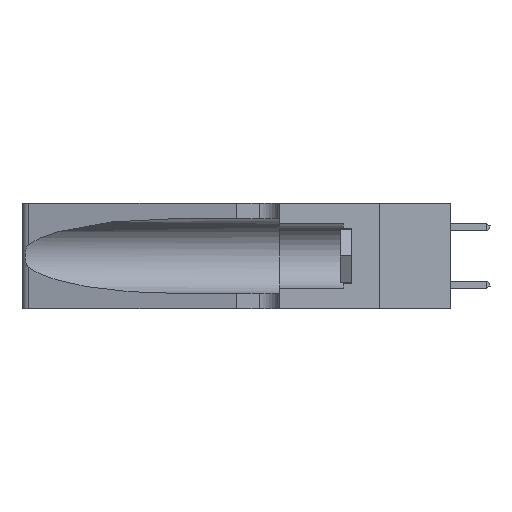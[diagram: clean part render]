
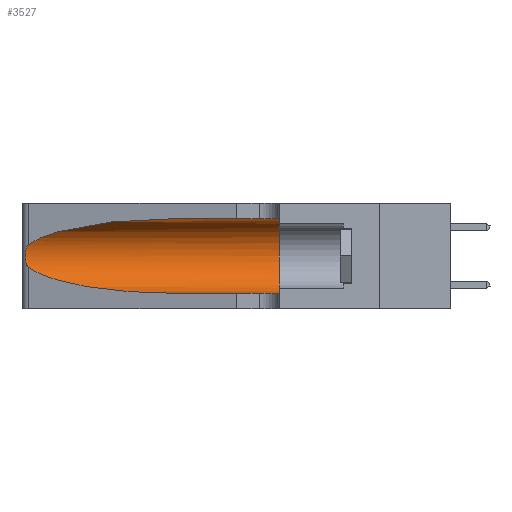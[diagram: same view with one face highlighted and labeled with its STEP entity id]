
A CAD part, left-side view. The second image highlights one B-rep face of the part: STEP entity #3527.
In plain terms, the highlighted cylindrical face has radius 3.308 mm (diameter 6.617 mm), a partial arc.
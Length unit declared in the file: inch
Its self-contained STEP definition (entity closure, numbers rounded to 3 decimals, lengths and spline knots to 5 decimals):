
#515 = EDGE_CURVE ( 'NONE', #18093, #35424, #3145, .T. ) ;
#1190 = ORIENTED_EDGE ( 'NONE', *, *, #40529, .T. ) ;
#1781 = CARTESIAN_POINT ( 'NONE',  ( 0.25639, 1.23184, 0.21858 ) ) ;
#3145 = CIRCLE ( 'NONE', #7678, 0.13025 ) ;
#3527 = ADVANCED_FACE ( 'NONE', ( #8425 ), #3908, .F. ) ;
#3906 = CARTESIAN_POINT ( 'NONE',  ( 0.2373, 1.15595, 0.28018 ) ) ;
#3908 = CYLINDRICAL_SURFACE ( 'NONE', #10126, 0.13025 ) ;
#4220 = CARTESIAN_POINT ( 'NONE',  ( 0.1305, 0.35, 0.05475 ) ) ;
#4902 = CARTESIAN_POINT ( 'NONE',  ( 0.25487, 1.22718, 0.14631 ) ) ;
#5651 = CARTESIAN_POINT ( 'NONE',  ( 0.1305, 0.72297, 0.05475 ) ) ;
#7044 = ORIENTED_EDGE ( 'NONE', *, *, #16871, .T. ) ;
#7301 = CARTESIAN_POINT ( 'NONE',  ( 0.18966, 0.96281, 0.31525 ) ) ;
#7351 = ORIENTED_EDGE ( 'NONE', *, *, #35953, .T. ) ;
#7678 = AXIS2_PLACEMENT_3D ( 'NONE', #40619, #15303, #31116 ) ;
#7974 = EDGE_LOOP ( 'NONE', ( #25872, #7351, #1190, #7044, #30697, #40650 ) ) ;
#8233 = CARTESIAN_POINT ( 'NONE',  ( 0.25854, 1.2359, 0.20912 ) ) ;
#8376 = CARTESIAN_POINT ( 'NONE',  ( 0.25789, 1.23486, 0.15765 ) ) ;
#8425 = FACE_OUTER_BOUND ( 'NONE', #7974, .T. ) ;
#8878 = CARTESIAN_POINT ( 'NONE',  ( 0.1305, 1.61858, 0.185 ) ) ;
#9000 = CARTESIAN_POINT ( 'NONE',  ( 0.1305, 1.61858, 0.05475 ) ) ;
#10126 = AXIS2_PLACEMENT_3D ( 'NONE', #8878, #20438, #39386 ) ;
#11963 = CARTESIAN_POINT ( 'NONE',  ( 0.25487, 1.22718, 0.14631 ) ) ;
#12708 =( BOUNDED_CURVE ( )  B_SPLINE_CURVE ( 3, ( #11963, #34762, #18709, #5651 ),
 .UNSPECIFIED., .F., .F. ) 
 B_SPLINE_CURVE_WITH_KNOTS ( ( 4, 4 ),
 ( 3.44316, 4.71239 ),
 .UNSPECIFIED. ) 
 CURVE ( )  GEOMETRIC_REPRESENTATION_ITEM ( )  RATIONAL_B_SPLINE_CURVE ( ( 1., 0.87, 0.87, 1. ) ) 
 REPRESENTATION_ITEM ( '' )  );
#14700 = CARTESIAN_POINT ( 'NONE',  ( 0.25787, 1.23484, 0.2124 ) ) ;
#15303 = DIRECTION ( 'NONE',  ( 0., 1., 0. ) ) ;
#15795 = B_SPLINE_CURVE_WITH_KNOTS ( 'NONE', 3,
 ( #23760, #30765, #1781, #14700, #8233, #17822, #34158, #24302, #40429, #33868, #8376, #33738, #31067, #4902 ),
 .UNSPECIFIED., .F., .F.,
 ( 4, 2, 2, 2, 2, 2, 4 ),
 ( 0., 0.00027, 0.00053, 0.00107, 0.0016, 0.00187, 0.00214 ),
 .UNSPECIFIED. ) ;
#16848 = VECTOR ( 'NONE', #28406, 39.37008 ) ;
#16871 = EDGE_CURVE ( 'NONE', #28863, #35424, #31520, .T. ) ;
#17822 = CARTESIAN_POINT ( 'NONE',  ( 0.26018, 1.23835, 0.19895 ) ) ;
#18093 = VERTEX_POINT ( 'NONE', #35486 ) ;
#18350 = VECTOR ( 'NONE', #19617, 39.37008 ) ;
#18709 = CARTESIAN_POINT ( 'NONE',  ( 0.18966, 0.96281, 0.05475 ) ) ;
#19617 = DIRECTION ( 'NONE',  ( 0., -1., 0. ) ) ;
#20438 = DIRECTION ( 'NONE',  ( 0., -1., 0. ) ) ;
#23319 =( BOUNDED_CURVE ( )  B_SPLINE_CURVE ( 3, ( #33464, #7301, #3906, #30061 ),
 .UNSPECIFIED., .F., .F. ) 
 B_SPLINE_CURVE_WITH_KNOTS ( ( 4, 4 ),
 ( 1.5708, 2.84003 ),
 .UNSPECIFIED. ) 
 CURVE ( )  GEOMETRIC_REPRESENTATION_ITEM ( )  RATIONAL_B_SPLINE_CURVE ( ( 1., 0.87, 0.87, 1. ) ) 
 REPRESENTATION_ITEM ( '' )  );
#23760 = CARTESIAN_POINT ( 'NONE',  ( 0.25487, 1.22718, 0.22369 ) ) ;
#24302 = CARTESIAN_POINT ( 'NONE',  ( 0.26075, 1.23896, 0.178 ) ) ;
#24686 = EDGE_CURVE ( 'NONE', #25807, #27607, #23319, .T. ) ;
#25807 = VERTEX_POINT ( 'NONE', #30289 ) ;
#25872 = ORIENTED_EDGE ( 'NONE', *, *, #24686, .T. ) ;
#27607 = VERTEX_POINT ( 'NONE', #36550 ) ;
#27954 = LINE ( 'NONE', #38890, #18350 ) ;
#28406 = DIRECTION ( 'NONE',  ( 0., -1., 0. ) ) ;
#28863 = VERTEX_POINT ( 'NONE', #36053 ) ;
#30061 = CARTESIAN_POINT ( 'NONE',  ( 0.25487, 1.22718, 0.22369 ) ) ;
#30289 = CARTESIAN_POINT ( 'NONE',  ( 0.1305, 0.72297, 0.31525 ) ) ;
#30697 = ORIENTED_EDGE ( 'NONE', *, *, #515, .F. ) ;
#30765 = CARTESIAN_POINT ( 'NONE',  ( 0.25555, 1.22994, 0.2215 ) ) ;
#31067 = CARTESIAN_POINT ( 'NONE',  ( 0.25555, 1.22993, 0.14849 ) ) ;
#31116 = DIRECTION ( 'NONE',  ( 0., 0., 1. ) ) ;
#31520 = LINE ( 'NONE', #9000, #16848 ) ;
#31763 = CARTESIAN_POINT ( 'NONE',  ( 0.25487, 1.22718, 0.14631 ) ) ;
#33464 = CARTESIAN_POINT ( 'NONE',  ( 0.1305, 0.72297, 0.31525 ) ) ;
#33738 = CARTESIAN_POINT ( 'NONE',  ( 0.25639, 1.23186, 0.15144 ) ) ;
#33868 = CARTESIAN_POINT ( 'NONE',  ( 0.25856, 1.23593, 0.16098 ) ) ;
#34158 = CARTESIAN_POINT ( 'NONE',  ( 0.26075, 1.23896, 0.19203 ) ) ;
#34762 = CARTESIAN_POINT ( 'NONE',  ( 0.2373, 1.15595, 0.08982 ) ) ;
#35424 = VERTEX_POINT ( 'NONE', #4220 ) ;
#35486 = CARTESIAN_POINT ( 'NONE',  ( 0.1305, 0.35, 0.31525 ) ) ;
#35953 = EDGE_CURVE ( 'NONE', #27607, #36223, #15795, .T. ) ;
#36053 = CARTESIAN_POINT ( 'NONE',  ( 0.1305, 0.72297, 0.05475 ) ) ;
#36223 = VERTEX_POINT ( 'NONE', #31763 ) ;
#36550 = CARTESIAN_POINT ( 'NONE',  ( 0.25487, 1.22718, 0.22369 ) ) ;
#38890 = CARTESIAN_POINT ( 'NONE',  ( 0.1305, 1.61858, 0.31525 ) ) ;
#39360 = EDGE_CURVE ( 'NONE', #25807, #18093, #27954, .T. ) ;
#39386 = DIRECTION ( 'NONE',  ( 0., 0., -1. ) ) ;
#40429 = CARTESIAN_POINT ( 'NONE',  ( 0.26017, 1.23833, 0.17102 ) ) ;
#40529 = EDGE_CURVE ( 'NONE', #36223, #28863, #12708, .T. ) ;
#40619 = CARTESIAN_POINT ( 'NONE',  ( 0.1305, 0.35, 0.185 ) ) ;
#40650 = ORIENTED_EDGE ( 'NONE', *, *, #39360, .F. ) ;
